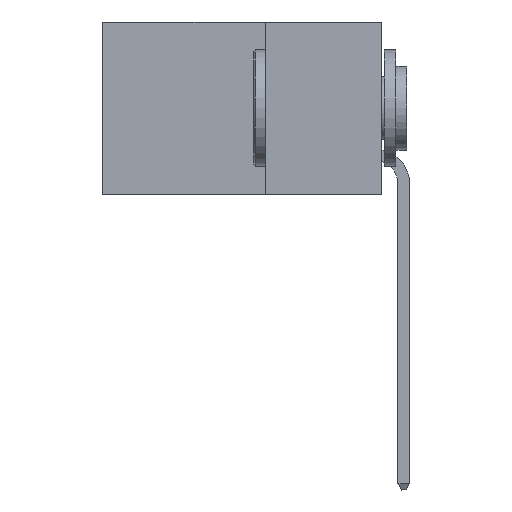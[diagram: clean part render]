
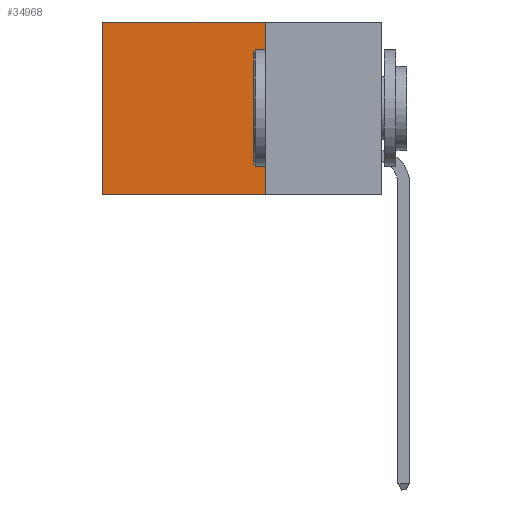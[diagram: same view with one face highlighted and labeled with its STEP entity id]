
A CAD part, left-side view. The second image highlights one B-rep face of the part: STEP entity #34968.
In plain terms, the highlighted planar face has unit normal (-1, 0, 0).
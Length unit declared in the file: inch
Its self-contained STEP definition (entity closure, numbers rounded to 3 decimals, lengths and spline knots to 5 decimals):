
#2072 = AXIS2_PLACEMENT_3D ( 'NONE', #31600, #8810, #34970 ) ;
#2226 = ORIENTED_EDGE ( 'NONE', *, *, #42624, .T. ) ;
#2553 = CARTESIAN_POINT ( 'NONE',  ( 0.2875, 0.25, 0. ) ) ;
#3448 = EDGE_CURVE ( 'NONE', #31010, #19738, #22024, .T. ) ;
#5201 = EDGE_LOOP ( 'NONE', ( #35642, #23454, #29756, #2226 ) ) ;
#5446 = LINE ( 'NONE', #12650, #16543 ) ;
#5563 = CARTESIAN_POINT ( 'NONE',  ( 0.2875, 0.6, -0.37 ) ) ;
#6788 = CARTESIAN_POINT ( 'NONE',  ( 0.2875, 0.6, 0. ) ) ;
#8518 = VERTEX_POINT ( 'NONE', #36786 ) ;
#8810 = DIRECTION ( 'NONE',  ( 1., 0., 0. ) ) ;
#12650 = CARTESIAN_POINT ( 'NONE',  ( 0.2875, 0.25, -0.37 ) ) ;
#13685 = DIRECTION ( 'NONE',  ( 0., 0., -1. ) ) ;
#14569 = LINE ( 'NONE', #17447, #30860 ) ;
#16543 = VECTOR ( 'NONE', #38583, 39.37008 ) ;
#17447 = CARTESIAN_POINT ( 'NONE',  ( 0.2875, 0.25, 0. ) ) ;
#17873 = EDGE_CURVE ( 'NONE', #25933, #8518, #14569, .T. ) ;
#18747 = VECTOR ( 'NONE', #40102, 39.37008 ) ;
#19738 = VERTEX_POINT ( 'NONE', #5563 ) ;
#20267 = PLANE ( 'NONE',  #2072 ) ;
#22024 = LINE ( 'NONE', #27736, #30091 ) ;
#23454 = ORIENTED_EDGE ( 'NONE', *, *, #26722, .F. ) ;
#25245 = LINE ( 'NONE', #2553, #18747 ) ;
#25933 = VERTEX_POINT ( 'NONE', #41924 ) ;
#26722 = EDGE_CURVE ( 'NONE', #8518, #19738, #5446, .T. ) ;
#27736 = CARTESIAN_POINT ( 'NONE',  ( 0.2875, 0.6, 0. ) ) ;
#29756 = ORIENTED_EDGE ( 'NONE', *, *, #17873, .F. ) ;
#30091 = VECTOR ( 'NONE', #35727, 39.37008 ) ;
#30860 = VECTOR ( 'NONE', #13685, 39.37008 ) ;
#31010 = VERTEX_POINT ( 'NONE', #6788 ) ;
#31600 = CARTESIAN_POINT ( 'NONE',  ( 0.2875, 0.25, 0. ) ) ;
#34968 = ADVANCED_FACE ( 'NONE', ( #42301 ), #20267, .F. ) ;
#34970 = DIRECTION ( 'NONE',  ( 0., 0., -1. ) ) ;
#35642 = ORIENTED_EDGE ( 'NONE', *, *, #3448, .T. ) ;
#35727 = DIRECTION ( 'NONE',  ( 0., 0., -1. ) ) ;
#36786 = CARTESIAN_POINT ( 'NONE',  ( 0.2875, 0.25, -0.37 ) ) ;
#38583 = DIRECTION ( 'NONE',  ( 0., 1., 0. ) ) ;
#40102 = DIRECTION ( 'NONE',  ( 0., 1., 0. ) ) ;
#41924 = CARTESIAN_POINT ( 'NONE',  ( 0.2875, 0.25, 0. ) ) ;
#42301 = FACE_OUTER_BOUND ( 'NONE', #5201, .T. ) ;
#42624 = EDGE_CURVE ( 'NONE', #25933, #31010, #25245, .T. ) ;
